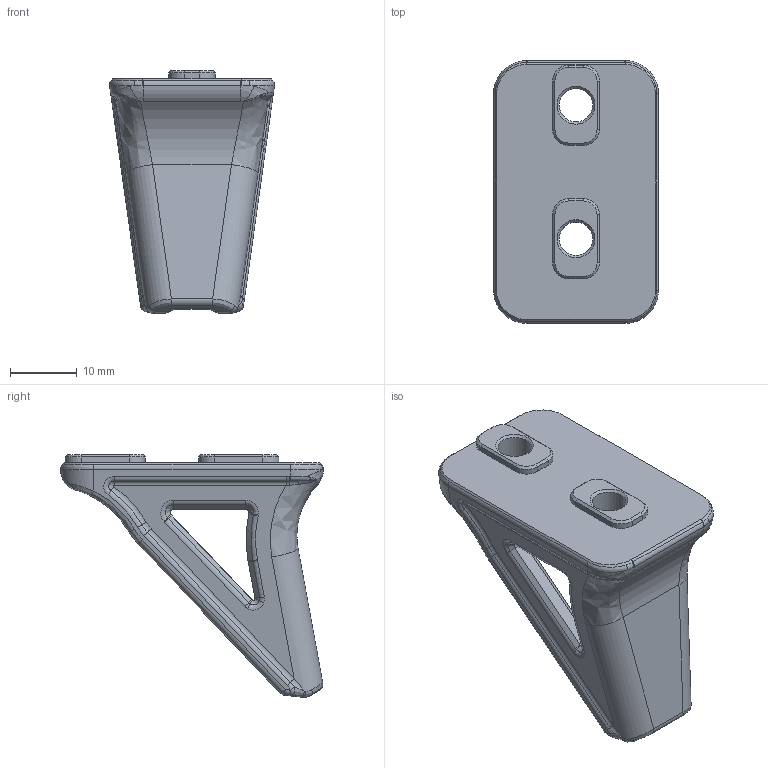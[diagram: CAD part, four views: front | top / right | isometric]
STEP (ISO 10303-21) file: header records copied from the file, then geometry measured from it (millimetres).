
FILE_DESCRIPTION(/* description */ (''),/* implementation_level */ '2;1');
FILE_NAME(/* name */ 'Standard.step',/* time_stamp */ '2021-07-02T17:40:44-04:00',/* author */ (''),/* organization */ (''),/* preprocessor_version */ 'ST-DEVELOPER v18.1',/* originating_system */ 'Autodesk Translation Framework v10.9.0.1377',/* authorisation */ '');
FILE_SCHEMA (('AUTOMOTIVE_DESIGN { 1 0 10303 214 3 1 1 }'));
Length unit declared in the file: millimetre
Products named in the file (1): Untitled
Bounding box: 24.72 x 39.39 x 36.36 mm (x, y, z)
Volume: 8088.9 mm3; surface area: 5039.6 mm2
Topology: 1 solids, 1 shells, 346 faces, 821 edges, 471 vertices
Faces by surface type: bspline 202, cylinder 69, plane 59, cone 10, sphere 6
Full cylindrical faces by diameter (mm): 5 x2
Entity records: 13852 total; most frequent: CARTESIAN_POINT 6989, ORIENTED_EDGE 1626, DIRECTION 1042, EDGE_CURVE 813, VERTEX_POINT 471, AXIS2_PLACEMENT_3D 392, EDGE_LOOP 356, FACE_OUTER_BOUND 346
